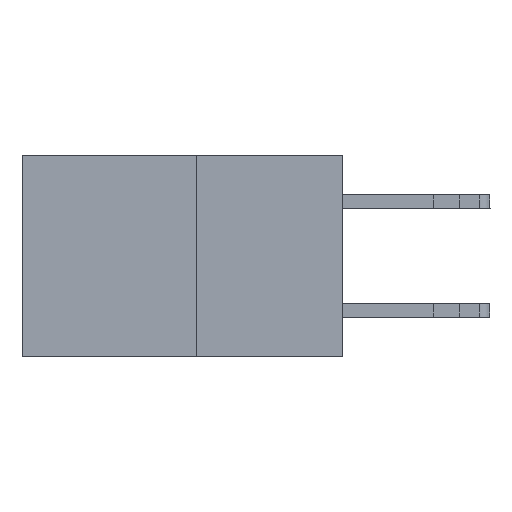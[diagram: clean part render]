
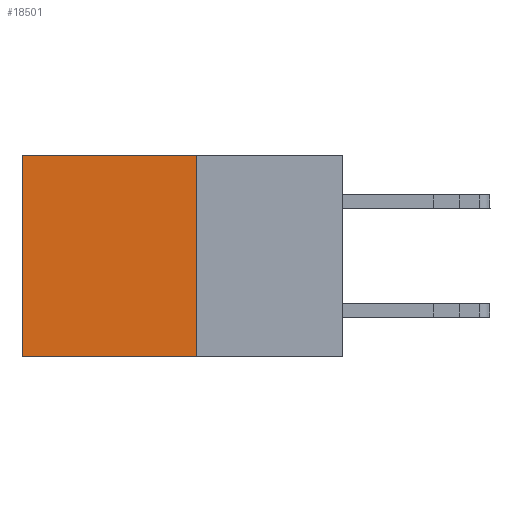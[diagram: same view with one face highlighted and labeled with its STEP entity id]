
A CAD part, left-side view. The second image highlights one B-rep face of the part: STEP entity #18501.
In plain terms, the highlighted planar face has unit normal (-1, 0, 0).
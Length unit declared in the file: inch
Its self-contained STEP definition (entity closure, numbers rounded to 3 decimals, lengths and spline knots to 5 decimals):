
#68 = CARTESIAN_POINT ( 'NONE',  ( 0.277, 0.59, -0.37 ) ) ;
#95 = VECTOR ( 'NONE', #352, 39.37008 ) ;
#352 = DIRECTION ( 'NONE',  ( 0., 0., -1. ) ) ;
#1319 = DIRECTION ( 'NONE',  ( 0., 0., -1. ) ) ;
#1767 = EDGE_CURVE ( 'NONE', #5980, #11332, #10805, .T. ) ;
#2155 = EDGE_LOOP ( 'NONE', ( #13812, #6521, #7424, #16364 ) ) ;
#3081 = EDGE_CURVE ( 'NONE', #7799, #11332, #8583, .T. ) ;
#3316 = CARTESIAN_POINT ( 'NONE',  ( 0.277, 0.27, 0. ) ) ;
#3437 = VECTOR ( 'NONE', #7392, 39.37008 ) ;
#4515 = LINE ( 'NONE', #3316, #16549 ) ;
#4779 = PLANE ( 'NONE',  #13541 ) ;
#5980 = VERTEX_POINT ( 'NONE', #17237 ) ;
#6384 = CARTESIAN_POINT ( 'NONE',  ( 0.277, 0.27, -0.37 ) ) ;
#6521 = ORIENTED_EDGE ( 'NONE', *, *, #1767, .F. ) ;
#6915 = LINE ( 'NONE', #20098, #14786 ) ;
#7392 = DIRECTION ( 'NONE',  ( 0., 1., 0. ) ) ;
#7424 = ORIENTED_EDGE ( 'NONE', *, *, #15943, .F. ) ;
#7799 = VERTEX_POINT ( 'NONE', #14228 ) ;
#7983 = DIRECTION ( 'NONE',  ( 1., 0., 0. ) ) ;
#8552 = FACE_OUTER_BOUND ( 'NONE', #2155, .T. ) ;
#8583 = LINE ( 'NONE', #68, #95 ) ;
#8636 = CARTESIAN_POINT ( 'NONE',  ( 0.277, 0.27, -0.37 ) ) ;
#10805 = LINE ( 'NONE', #8636, #3437 ) ;
#11332 = VERTEX_POINT ( 'NONE', #16249 ) ;
#13541 = AXIS2_PLACEMENT_3D ( 'NONE', #6384, #7983, #18838 ) ;
#13635 = CARTESIAN_POINT ( 'NONE',  ( 0.277, 0.27, 0. ) ) ;
#13812 = ORIENTED_EDGE ( 'NONE', *, *, #3081, .T. ) ;
#14228 = CARTESIAN_POINT ( 'NONE',  ( 0.277, 0.59, 0. ) ) ;
#14786 = VECTOR ( 'NONE', #1319, 39.37008 ) ;
#15943 = EDGE_CURVE ( 'NONE', #20301, #5980, #6915, .T. ) ;
#15949 = DIRECTION ( 'NONE',  ( 0., 1., 0. ) ) ;
#16249 = CARTESIAN_POINT ( 'NONE',  ( 0.277, 0.59, -0.37 ) ) ;
#16364 = ORIENTED_EDGE ( 'NONE', *, *, #19951, .T. ) ;
#16549 = VECTOR ( 'NONE', #15949, 39.37008 ) ;
#17237 = CARTESIAN_POINT ( 'NONE',  ( 0.277, 0.27, -0.37 ) ) ;
#18501 = ADVANCED_FACE ( 'NONE', ( #8552 ), #4779, .F. ) ;
#18838 = DIRECTION ( 'NONE',  ( 0., 0., -1. ) ) ;
#19951 = EDGE_CURVE ( 'NONE', #20301, #7799, #4515, .T. ) ;
#20098 = CARTESIAN_POINT ( 'NONE',  ( 0.277, 0.27, -0.37 ) ) ;
#20301 = VERTEX_POINT ( 'NONE', #13635 ) ;
